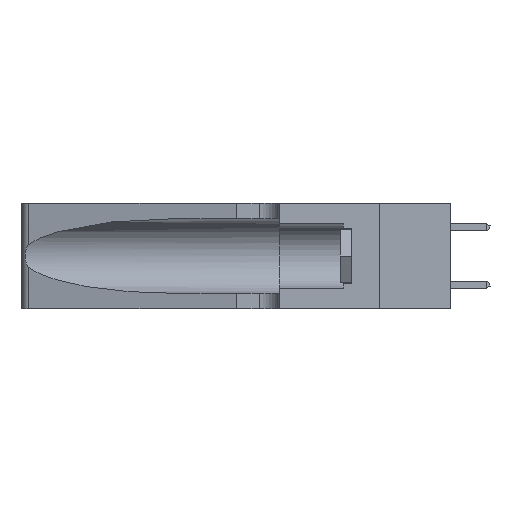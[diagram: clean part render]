
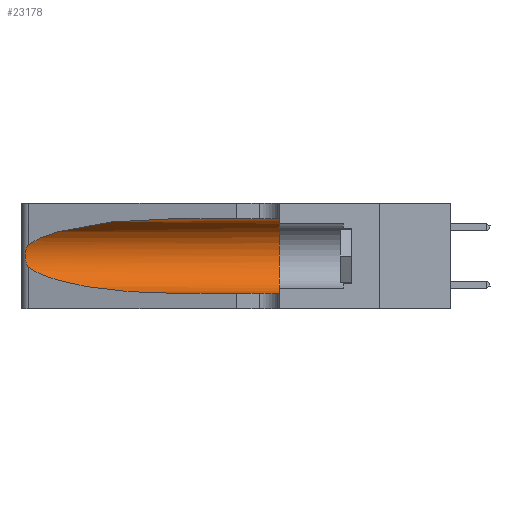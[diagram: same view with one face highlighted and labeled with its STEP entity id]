
A CAD part, left-side view. The second image highlights one B-rep face of the part: STEP entity #23178.
In plain terms, the highlighted cylindrical face has radius 3.308 mm (diameter 6.617 mm), a partial arc.
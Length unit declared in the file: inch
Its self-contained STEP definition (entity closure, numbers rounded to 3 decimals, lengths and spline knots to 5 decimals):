
#320 = DIRECTION ( 'NONE',  ( 0., -1., 0. ) ) ;
#487 = ORIENTED_EDGE ( 'NONE', *, *, #4966, .T. ) ;
#1351 = CARTESIAN_POINT ( 'NONE',  ( 0.25555, 1.22994, 0.2215 ) ) ;
#1459 = EDGE_CURVE ( 'NONE', #23092, #18468, #8312, .T. ) ;
#1469 = CARTESIAN_POINT ( 'NONE',  ( 0.26075, 1.23896, 0.178 ) ) ;
#1795 = ORIENTED_EDGE ( 'NONE', *, *, #6500, .F. ) ;
#2881 = EDGE_CURVE ( 'NONE', #13161, #23092, #11082, .T. ) ;
#3864 = CARTESIAN_POINT ( 'NONE',  ( 0.25856, 1.23593, 0.16098 ) ) ;
#4966 = EDGE_CURVE ( 'NONE', #23507, #13161, #15819, .T. ) ;
#5052 = CARTESIAN_POINT ( 'NONE',  ( 0.1305, 0.35, 0.05475 ) ) ;
#5600 = CARTESIAN_POINT ( 'NONE',  ( 0.2373, 1.15595, 0.08982 ) ) ;
#5721 = CARTESIAN_POINT ( 'NONE',  ( 0.1305, 0.72297, 0.05475 ) ) ;
#6500 = EDGE_CURVE ( 'NONE', #23507, #24874, #10060, .T. ) ;
#6833 = EDGE_CURVE ( 'NONE', #24874, #17908, #25567, .T. ) ;
#6918 = DIRECTION ( 'NONE',  ( 0., 0., -1. ) ) ;
#7581 = AXIS2_PLACEMENT_3D ( 'NONE', #13872, #20625, #10981 ) ;
#8180 = CARTESIAN_POINT ( 'NONE',  ( 0.1305, 0.72297, 0.31525 ) ) ;
#8312 =( BOUNDED_CURVE ( )  B_SPLINE_CURVE ( 3, ( #10084, #5600, #23827, #5721 ),
 .UNSPECIFIED., .F., .F. ) 
 B_SPLINE_CURVE_WITH_KNOTS ( ( 4, 4 ),
 ( 3.44316, 4.71239 ),
 .UNSPECIFIED. ) 
 CURVE ( )  GEOMETRIC_REPRESENTATION_ITEM ( )  RATIONAL_B_SPLINE_CURVE ( ( 1., 0.87, 0.87, 1. ) ) 
 REPRESENTATION_ITEM ( '' )  );
#8789 = EDGE_LOOP ( 'NONE', ( #487, #9791, #21363, #11570, #22370, #1795 ) ) ;
#8851 = CARTESIAN_POINT ( 'NONE',  ( 0.18966, 0.96281, 0.31525 ) ) ;
#9624 = FACE_OUTER_BOUND ( 'NONE', #8789, .T. ) ;
#9791 = ORIENTED_EDGE ( 'NONE', *, *, #2881, .T. ) ;
#10060 = LINE ( 'NONE', #11711, #21019 ) ;
#10084 = CARTESIAN_POINT ( 'NONE',  ( 0.25487, 1.22718, 0.14631 ) ) ;
#10764 = CARTESIAN_POINT ( 'NONE',  ( 0.25639, 1.23186, 0.15144 ) ) ;
#10957 = CARTESIAN_POINT ( 'NONE',  ( 0.26017, 1.23833, 0.17102 ) ) ;
#10981 = DIRECTION ( 'NONE',  ( 0., 0., 1. ) ) ;
#11082 = B_SPLINE_CURVE_WITH_KNOTS ( 'NONE', 3,
 ( #21806, #1351, #12622, #23863, #15225, #24065, #22002, #1469, #10957, #3864, #22098, #10764, #28779, #26705 ),
 .UNSPECIFIED., .F., .F.,
 ( 4, 2, 2, 2, 2, 2, 4 ),
 ( 0., 0.00027, 0.00053, 0.00107, 0.0016, 0.00187, 0.00214 ),
 .UNSPECIFIED. ) ;
#11570 = ORIENTED_EDGE ( 'NONE', *, *, #11668, .T. ) ;
#11668 = EDGE_CURVE ( 'NONE', #18468, #17908, #18275, .T. ) ;
#11711 = CARTESIAN_POINT ( 'NONE',  ( 0.1305, 1.61858, 0.31525 ) ) ;
#12622 = CARTESIAN_POINT ( 'NONE',  ( 0.25639, 1.23184, 0.21858 ) ) ;
#13161 = VERTEX_POINT ( 'NONE', #21179 ) ;
#13528 = CARTESIAN_POINT ( 'NONE',  ( 0.1305, 0.72297, 0.05475 ) ) ;
#13872 = CARTESIAN_POINT ( 'NONE',  ( 0.1305, 0.35, 0.185 ) ) ;
#14753 = VECTOR ( 'NONE', #18739, 39.37008 ) ;
#15225 = CARTESIAN_POINT ( 'NONE',  ( 0.25854, 1.2359, 0.20912 ) ) ;
#15690 = CYLINDRICAL_SURFACE ( 'NONE', #22665, 0.13025 ) ;
#15819 =( BOUNDED_CURVE ( )  B_SPLINE_CURVE ( 3, ( #29069, #8851, #26988, #20034 ),
 .UNSPECIFIED., .F., .T. ) 
 B_SPLINE_CURVE_WITH_KNOTS ( ( 4, 4 ),
 ( 1.5708, 2.84003 ),
 .UNSPECIFIED. ) 
 CURVE ( )  GEOMETRIC_REPRESENTATION_ITEM ( )  RATIONAL_B_SPLINE_CURVE ( ( 1., 0.87, 0.87, 1. ) ) 
 REPRESENTATION_ITEM ( '' )  );
#16216 = CARTESIAN_POINT ( 'NONE',  ( 0.1305, 1.61858, 0.05475 ) ) ;
#17908 = VERTEX_POINT ( 'NONE', #5052 ) ;
#18275 = LINE ( 'NONE', #16216, #14753 ) ;
#18468 = VERTEX_POINT ( 'NONE', #13528 ) ;
#18739 = DIRECTION ( 'NONE',  ( 0., -1., 0. ) ) ;
#20034 = CARTESIAN_POINT ( 'NONE',  ( 0.25487, 1.22718, 0.22369 ) ) ;
#20625 = DIRECTION ( 'NONE',  ( 0., 1., 0. ) ) ;
#21019 = VECTOR ( 'NONE', #320, 39.37008 ) ;
#21179 = CARTESIAN_POINT ( 'NONE',  ( 0.25487, 1.22718, 0.22369 ) ) ;
#21363 = ORIENTED_EDGE ( 'NONE', *, *, #1459, .T. ) ;
#21806 = CARTESIAN_POINT ( 'NONE',  ( 0.25487, 1.22718, 0.22369 ) ) ;
#21888 = CARTESIAN_POINT ( 'NONE',  ( 0.1305, 1.61858, 0.185 ) ) ;
#22002 = CARTESIAN_POINT ( 'NONE',  ( 0.26075, 1.23896, 0.19203 ) ) ;
#22098 = CARTESIAN_POINT ( 'NONE',  ( 0.25789, 1.23486, 0.15765 ) ) ;
#22156 = CARTESIAN_POINT ( 'NONE',  ( 0.1305, 0.35, 0.31525 ) ) ;
#22370 = ORIENTED_EDGE ( 'NONE', *, *, #6833, .F. ) ;
#22653 = DIRECTION ( 'NONE',  ( 0., -1., 0. ) ) ;
#22665 = AXIS2_PLACEMENT_3D ( 'NONE', #21888, #22653, #6918 ) ;
#23092 = VERTEX_POINT ( 'NONE', #26965 ) ;
#23178 = ADVANCED_FACE ( 'NONE', ( #9624 ), #15690, .F. ) ;
#23507 = VERTEX_POINT ( 'NONE', #8180 ) ;
#23827 = CARTESIAN_POINT ( 'NONE',  ( 0.18966, 0.96281, 0.05475 ) ) ;
#23863 = CARTESIAN_POINT ( 'NONE',  ( 0.25787, 1.23484, 0.2124 ) ) ;
#24065 = CARTESIAN_POINT ( 'NONE',  ( 0.26018, 1.23835, 0.19895 ) ) ;
#24874 = VERTEX_POINT ( 'NONE', #22156 ) ;
#25567 = CIRCLE ( 'NONE', #7581, 0.13025 ) ;
#26705 = CARTESIAN_POINT ( 'NONE',  ( 0.25487, 1.22718, 0.14631 ) ) ;
#26965 = CARTESIAN_POINT ( 'NONE',  ( 0.25487, 1.22718, 0.14631 ) ) ;
#26988 = CARTESIAN_POINT ( 'NONE',  ( 0.2373, 1.15595, 0.28018 ) ) ;
#28779 = CARTESIAN_POINT ( 'NONE',  ( 0.25555, 1.22993, 0.14849 ) ) ;
#29069 = CARTESIAN_POINT ( 'NONE',  ( 0.1305, 0.72297, 0.31525 ) ) ;
